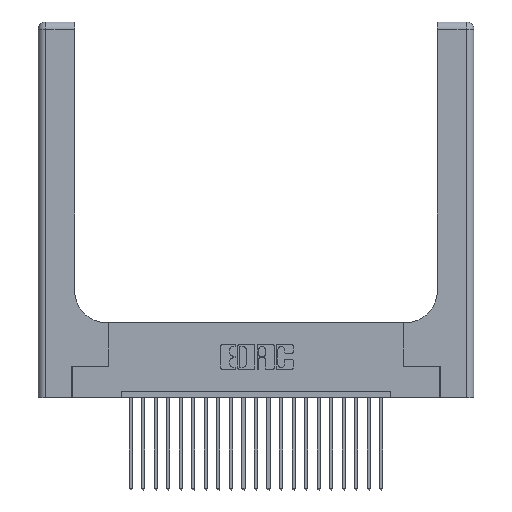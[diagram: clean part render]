
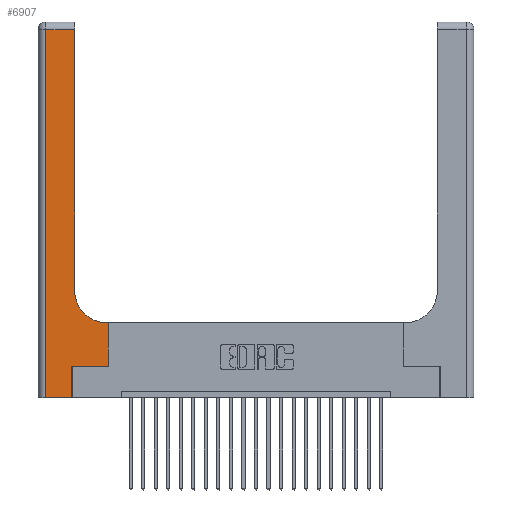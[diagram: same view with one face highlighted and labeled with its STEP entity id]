
A CAD part, top view. The second image highlights one B-rep face of the part: STEP entity #6907.
In plain terms, the highlighted planar face has unit normal (0, 0, 1).
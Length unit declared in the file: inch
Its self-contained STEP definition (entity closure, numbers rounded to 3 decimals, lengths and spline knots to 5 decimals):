
#925 = AXIS2_PLACEMENT_3D ( 'NONE', #14265, #3242, #18021 ) ;
#1227 = DIRECTION ( 'NONE',  ( 1., 0., 0. ) ) ;
#1299 = EDGE_CURVE ( 'NONE', #2119, #21282, #1935, .T. ) ;
#1346 = DIRECTION ( 'NONE',  ( 0., 0., -1. ) ) ;
#1660 = VERTEX_POINT ( 'NONE', #9250 ) ;
#1935 = CIRCLE ( 'NONE', #925, 0.25 ) ;
#2119 = VERTEX_POINT ( 'NONE', #20248 ) ;
#2186 = LINE ( 'NONE', #17617, #7671 ) ;
#3112 = VERTEX_POINT ( 'NONE', #11545 ) ;
#3131 = DIRECTION ( 'NONE',  ( -1., 0., 0. ) ) ;
#3242 = DIRECTION ( 'NONE',  ( 0., 0., -1. ) ) ;
#3294 = PLANE ( 'NONE',  #8164 ) ;
#3334 = CARTESIAN_POINT ( 'NONE',  ( 0.06, 2.94, 0.37 ) ) ;
#3517 = ORIENTED_EDGE ( 'NONE', *, *, #1299, .T. ) ;
#3543 = VECTOR ( 'NONE', #1227, 39.37008 ) ;
#3861 = CARTESIAN_POINT ( 'NONE',  ( 0.2915, 2.94, 0.37 ) ) ;
#4305 = CARTESIAN_POINT ( 'NONE',  ( 0.5585, 0.6, 0.37 ) ) ;
#4308 = VECTOR ( 'NONE', #14108, 39.37008 ) ;
#5135 = EDGE_CURVE ( 'NONE', #1660, #7703, #11011, .T. ) ;
#5856 = DIRECTION ( 'NONE',  ( 0., 1., 0. ) ) ;
#6026 = LINE ( 'NONE', #8398, #4308 ) ;
#6617 = LINE ( 'NONE', #10976, #23010 ) ;
#6688 = ORIENTED_EDGE ( 'NONE', *, *, #15377, .T. ) ;
#6907 = ADVANCED_FACE ( 'NONE', ( #9175 ), #3294, .F. ) ;
#7373 = DIRECTION ( 'NONE',  ( 1., 0., 0. ) ) ;
#7671 = VECTOR ( 'NONE', #10186, 39.37008 ) ;
#7703 = VERTEX_POINT ( 'NONE', #10090 ) ;
#8017 = ORIENTED_EDGE ( 'NONE', *, *, #11191, .T. ) ;
#8164 = AXIS2_PLACEMENT_3D ( 'NONE', #12228, #1346, #3131 ) ;
#8398 = CARTESIAN_POINT ( 'NONE',  ( 0.2915, 3., 0.37 ) ) ;
#8494 = LINE ( 'NONE', #11409, #15728 ) ;
#8544 = EDGE_CURVE ( 'NONE', #18553, #2119, #6617, .T. ) ;
#8767 = ORIENTED_EDGE ( 'NONE', *, *, #5135, .T. ) ;
#9067 = LINE ( 'NONE', #12332, #22586 ) ;
#9175 = FACE_OUTER_BOUND ( 'NONE', #13858, .T. ) ;
#9250 = CARTESIAN_POINT ( 'NONE',  ( 0.269, 0., 0.37 ) ) ;
#10090 = CARTESIAN_POINT ( 'NONE',  ( 0.269, 0.25, 0.37 ) ) ;
#10123 = VERTEX_POINT ( 'NONE', #3861 ) ;
#10186 = DIRECTION ( 'NONE',  ( 0., 1., 0. ) ) ;
#10976 = CARTESIAN_POINT ( 'NONE',  ( 0.2915, 0.6, 0.37 ) ) ;
#11011 = LINE ( 'NONE', #20793, #22793 ) ;
#11191 = EDGE_CURVE ( 'NONE', #10123, #22023, #9067, .T. ) ;
#11409 = CARTESIAN_POINT ( 'NONE',  ( 0.269, 0.25, 0.37 ) ) ;
#11545 = CARTESIAN_POINT ( 'NONE',  ( 0.5585, 0.25, 0.37 ) ) ;
#11640 = EDGE_CURVE ( 'NONE', #22023, #21651, #20618, .T. ) ;
#12228 = CARTESIAN_POINT ( 'NONE',  ( 0., 3., 0.37 ) ) ;
#12279 = EDGE_CURVE ( 'NONE', #21651, #1660, #17977, .T. ) ;
#12332 = CARTESIAN_POINT ( 'NONE',  ( 0., 2.94, 0.37 ) ) ;
#13290 = ORIENTED_EDGE ( 'NONE', *, *, #12279, .T. ) ;
#13627 = CARTESIAN_POINT ( 'NONE',  ( 0.06, 3., 0.37 ) ) ;
#13858 = EDGE_LOOP ( 'NONE', ( #15370, #8017, #19247, #13290, #8767, #19402, #6688, #18110, #3517 ) ) ;
#14108 = DIRECTION ( 'NONE',  ( 0., 1., 0. ) ) ;
#14265 = CARTESIAN_POINT ( 'NONE',  ( 0.5415, 0.85, 0.37 ) ) ;
#14491 = DIRECTION ( 'NONE',  ( -1., 0., 0. ) ) ;
#15370 = ORIENTED_EDGE ( 'NONE', *, *, #19999, .T. ) ;
#15377 = EDGE_CURVE ( 'NONE', #3112, #18553, #2186, .T. ) ;
#15728 = VECTOR ( 'NONE', #7373, 39.37008 ) ;
#16257 = VECTOR ( 'NONE', #17365, 39.37008 ) ;
#16521 = EDGE_CURVE ( 'NONE', #7703, #3112, #8494, .T. ) ;
#17365 = DIRECTION ( 'NONE',  ( 0., -1., 0. ) ) ;
#17617 = CARTESIAN_POINT ( 'NONE',  ( 0.5585, 0.25, 0.37 ) ) ;
#17977 = LINE ( 'NONE', #23201, #3543 ) ;
#18021 = DIRECTION ( 'NONE',  ( 1., 0., 0. ) ) ;
#18110 = ORIENTED_EDGE ( 'NONE', *, *, #8544, .T. ) ;
#18553 = VERTEX_POINT ( 'NONE', #4305 ) ;
#19247 = ORIENTED_EDGE ( 'NONE', *, *, #11640, .T. ) ;
#19402 = ORIENTED_EDGE ( 'NONE', *, *, #16521, .T. ) ;
#19999 = EDGE_CURVE ( 'NONE', #21282, #10123, #6026, .T. ) ;
#20248 = CARTESIAN_POINT ( 'NONE',  ( 0.5415, 0.6, 0.37 ) ) ;
#20618 = LINE ( 'NONE', #13627, #16257 ) ;
#20793 = CARTESIAN_POINT ( 'NONE',  ( 0.269, 0., 0.37 ) ) ;
#20959 = CARTESIAN_POINT ( 'NONE',  ( 0.06, 0., 0.37 ) ) ;
#21058 = CARTESIAN_POINT ( 'NONE',  ( 0.2915, 0.85, 0.37 ) ) ;
#21282 = VERTEX_POINT ( 'NONE', #21058 ) ;
#21651 = VERTEX_POINT ( 'NONE', #20959 ) ;
#21824 = DIRECTION ( 'NONE',  ( -1., 0., 0. ) ) ;
#22023 = VERTEX_POINT ( 'NONE', #3334 ) ;
#22586 = VECTOR ( 'NONE', #21824, 39.37008 ) ;
#22793 = VECTOR ( 'NONE', #5856, 39.37008 ) ;
#23010 = VECTOR ( 'NONE', #14491, 39.37008 ) ;
#23201 = CARTESIAN_POINT ( 'NONE',  ( 0., 0., 0.37 ) ) ;
